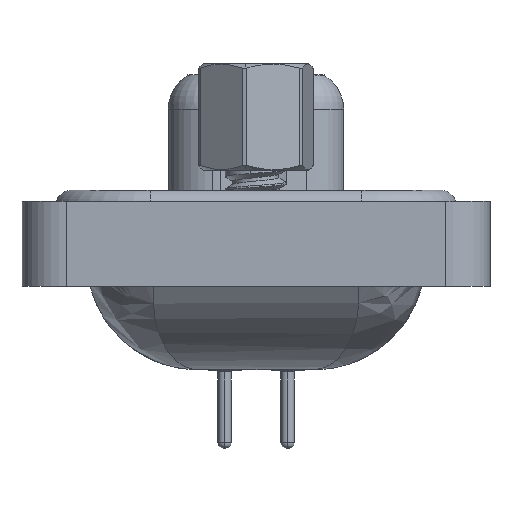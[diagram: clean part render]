
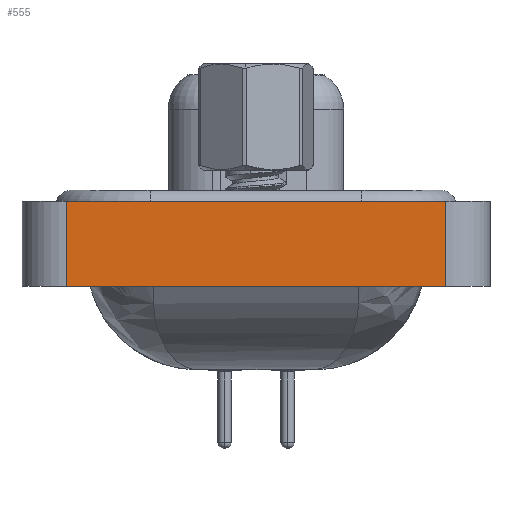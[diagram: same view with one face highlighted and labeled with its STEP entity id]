
A CAD part, left-side view. The second image highlights one B-rep face of the part: STEP entity #555.
In plain terms, the highlighted planar face has unit normal (-1, 0, 0).
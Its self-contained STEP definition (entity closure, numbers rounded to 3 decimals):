
#84 = LINE ( 'NONE', #20369, #12964 ) ;
#555 = ADVANCED_FACE ( 'NONE', ( #17217 ), #25896, .T. ) ;
#1275 = LINE ( 'NONE', #10385, #25600 ) ;
#1567 = VERTEX_POINT ( 'NONE', #11829 ) ;
#1854 = DIRECTION ( 'NONE',  ( 0., -1., 0. ) ) ;
#2494 = ORIENTED_EDGE ( 'NONE', *, *, #3358, .F. ) ;
#3124 = ORIENTED_EDGE ( 'NONE', *, *, #7060, .F. ) ;
#3247 = ORIENTED_EDGE ( 'NONE', *, *, #12027, .T. ) ;
#3358 = EDGE_CURVE ( 'NONE', #22974, #23499, #1275, .T. ) ;
#7060 = EDGE_CURVE ( 'NONE', #1567, #22974, #84, .T. ) ;
#9306 = EDGE_LOOP ( 'NONE', ( #3247, #2494, #3124, #17448 ) ) ;
#9498 = VECTOR ( 'NONE', #25423, 1000. ) ;
#10033 = DIRECTION ( 'NONE',  ( -1., 0., 0. ) ) ;
#10385 = CARTESIAN_POINT ( 'NONE',  ( -7.225, -8.55, 0.5 ) ) ;
#11829 = CARTESIAN_POINT ( 'NONE',  ( -7.225, 8.55, -3.35 ) ) ;
#12027 = EDGE_CURVE ( 'NONE', #13892, #23499, #14540, .T. ) ;
#12065 = CARTESIAN_POINT ( 'NONE',  ( -7.225, -8.55, -3.35 ) ) ;
#12307 = CARTESIAN_POINT ( 'NONE',  ( -7.225, 8.55, 0.5 ) ) ;
#12964 = VECTOR ( 'NONE', #22561, 1000. ) ;
#13892 = VERTEX_POINT ( 'NONE', #12065 ) ;
#14540 = LINE ( 'NONE', #16455, #9498 ) ;
#14866 = DIRECTION ( 'NONE',  ( 0., 0., 1. ) ) ;
#15290 = CARTESIAN_POINT ( 'NONE',  ( -7.225, -8.55, -3.35 ) ) ;
#16455 = CARTESIAN_POINT ( 'NONE',  ( -7.225, -8.55, -3.35 ) ) ;
#17217 = FACE_OUTER_BOUND ( 'NONE', #9306, .T. ) ;
#17448 = ORIENTED_EDGE ( 'NONE', *, *, #20729, .T. ) ;
#19751 = CARTESIAN_POINT ( 'NONE',  ( -7.225, -8.55, 0.5 ) ) ;
#20369 = CARTESIAN_POINT ( 'NONE',  ( -7.225, 8.55, -3.35 ) ) ;
#20444 = VECTOR ( 'NONE', #25779, 1000. ) ;
#20729 = EDGE_CURVE ( 'NONE', #1567, #13892, #22059, .T. ) ;
#21489 = CARTESIAN_POINT ( 'NONE',  ( -7.225, -8.55, -3.35 ) ) ;
#22059 = LINE ( 'NONE', #15290, #20444 ) ;
#22481 = AXIS2_PLACEMENT_3D ( 'NONE', #21489, #10033, #14866 ) ;
#22561 = DIRECTION ( 'NONE',  ( 0., 0., 1. ) ) ;
#22974 = VERTEX_POINT ( 'NONE', #12307 ) ;
#23499 = VERTEX_POINT ( 'NONE', #19751 ) ;
#25423 = DIRECTION ( 'NONE',  ( 0., 0., 1. ) ) ;
#25600 = VECTOR ( 'NONE', #1854, 1000. ) ;
#25779 = DIRECTION ( 'NONE',  ( 0., -1., 0. ) ) ;
#25896 = PLANE ( 'NONE',  #22481 ) ;
